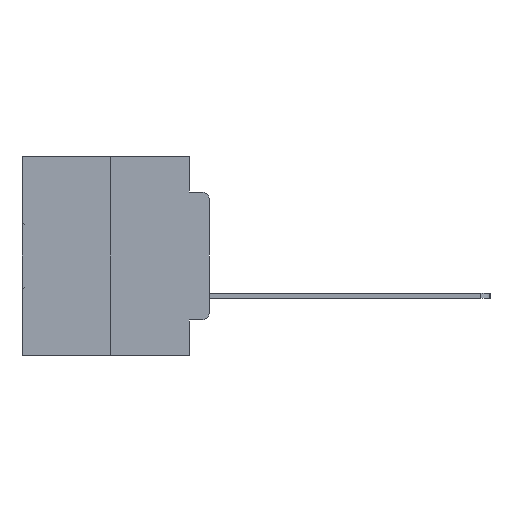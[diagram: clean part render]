
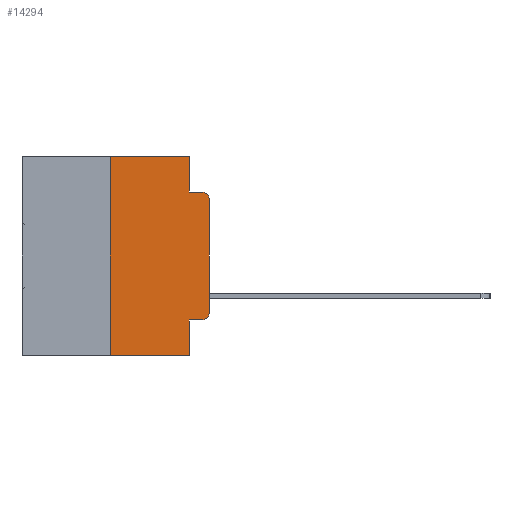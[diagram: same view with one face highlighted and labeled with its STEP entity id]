
A CAD part, left-side view. The second image highlights one B-rep face of the part: STEP entity #14294.
In plain terms, the highlighted planar face has unit normal (-1, 0, 0).
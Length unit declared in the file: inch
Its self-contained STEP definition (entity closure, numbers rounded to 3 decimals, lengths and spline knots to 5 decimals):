
#706 = ORIENTED_EDGE ( 'NONE', *, *, #26774, .F. ) ;
#952 = DIRECTION ( 'NONE',  ( 1., 0., 0. ) ) ;
#971 = LINE ( 'NONE', #20506, #6593 ) ;
#1657 = CARTESIAN_POINT ( 'NONE',  ( 0., 0.25, -0.5 ) ) ;
#2181 = ORIENTED_EDGE ( 'NONE', *, *, #8467, .T. ) ;
#2352 = LINE ( 'NONE', #14920, #7245 ) ;
#2568 = CARTESIAN_POINT ( 'NONE',  ( 0., 0.051, -0.0885 ) ) ;
#2713 = DIRECTION ( 'NONE',  ( -1., 0., 0. ) ) ;
#2879 = CARTESIAN_POINT ( 'NONE',  ( 0., 0., -0.3915 ) ) ;
#4045 = ORIENTED_EDGE ( 'NONE', *, *, #10219, .F. ) ;
#5011 = LINE ( 'NONE', #5101, #28665 ) ;
#5101 = CARTESIAN_POINT ( 'NONE',  ( 0., 0.051, 0. ) ) ;
#5233 = CARTESIAN_POINT ( 'NONE',  ( 0., 0.051, -0.4115 ) ) ;
#5458 = CARTESIAN_POINT ( 'NONE',  ( 0., 0.25, 0. ) ) ;
#6114 = VECTOR ( 'NONE', #24786, 39.37008 ) ;
#6127 = CARTESIAN_POINT ( 'NONE',  ( 0., 0.051, -0.5 ) ) ;
#6136 = CARTESIAN_POINT ( 'NONE',  ( 0., 0., -0.1085 ) ) ;
#6593 = VECTOR ( 'NONE', #22897, 39.37008 ) ;
#7245 = VECTOR ( 'NONE', #17186, 39.37008 ) ;
#7883 = DIRECTION ( 'NONE',  ( 0., 0., 1. ) ) ;
#8215 = VERTEX_POINT ( 'NONE', #1657 ) ;
#8255 = VERTEX_POINT ( 'NONE', #9101 ) ;
#8276 = VERTEX_POINT ( 'NONE', #27923 ) ;
#8467 = EDGE_CURVE ( 'NONE', #8215, #18024, #19952, .T. ) ;
#8807 = CIRCLE ( 'NONE', #24011, 0.02 ) ;
#8814 = CARTESIAN_POINT ( 'NONE',  ( 0., 0.473, 0. ) ) ;
#9101 = CARTESIAN_POINT ( 'NONE',  ( 0., 0.02, -0.0885 ) ) ;
#9537 = VECTOR ( 'NONE', #25926, 39.37008 ) ;
#10219 = EDGE_CURVE ( 'NONE', #8276, #28659, #19099, .T. ) ;
#11506 = DIRECTION ( 'NONE',  ( 0., -1., 0. ) ) ;
#12866 = CARTESIAN_POINT ( 'NONE',  ( 0., 0.473, 0. ) ) ;
#13652 = CARTESIAN_POINT ( 'NONE',  ( 0., 0.02, -0.1085 ) ) ;
#13888 = VERTEX_POINT ( 'NONE', #6136 ) ;
#13963 = LINE ( 'NONE', #17682, #6114 ) ;
#14103 = CARTESIAN_POINT ( 'NONE',  ( 0., 0.051, 0. ) ) ;
#14232 = VERTEX_POINT ( 'NONE', #26643 ) ;
#14294 = ADVANCED_FACE ( 'NONE', ( #25542 ), #22254, .F. ) ;
#14920 = CARTESIAN_POINT ( 'NONE',  ( 0., 0.051, -0.0885 ) ) ;
#15643 = EDGE_CURVE ( 'NONE', #21927, #14232, #971, .T. ) ;
#15954 = AXIS2_PLACEMENT_3D ( 'NONE', #12866, #952, #17613 ) ;
#15991 = ORIENTED_EDGE ( 'NONE', *, *, #20480, .F. ) ;
#16011 = DIRECTION ( 'NONE',  ( 0., 0., -1. ) ) ;
#16371 = ORIENTED_EDGE ( 'NONE', *, *, #16571, .F. ) ;
#16571 = EDGE_CURVE ( 'NONE', #21927, #18024, #5011, .T. ) ;
#16829 = CARTESIAN_POINT ( 'NONE',  ( 0., 0.051, 0. ) ) ;
#16968 = DIRECTION ( 'NONE',  ( 0., 0., -1. ) ) ;
#16992 = CARTESIAN_POINT ( 'NONE',  ( 0., 0.02, -0.3915 ) ) ;
#17083 = ORIENTED_EDGE ( 'NONE', *, *, #20782, .T. ) ;
#17186 = DIRECTION ( 'NONE',  ( 0., -1., 0. ) ) ;
#17613 = DIRECTION ( 'NONE',  ( 0., 0., -1. ) ) ;
#17682 = CARTESIAN_POINT ( 'NONE',  ( 0., 0., 0. ) ) ;
#17763 = VERTEX_POINT ( 'NONE', #2568 ) ;
#18024 = VERTEX_POINT ( 'NONE', #6127 ) ;
#18377 = VECTOR ( 'NONE', #23060, 39.37008 ) ;
#19099 = LINE ( 'NONE', #8814, #18377 ) ;
#19323 = DIRECTION ( 'NONE',  ( 0., 0., -1. ) ) ;
#19952 = LINE ( 'NONE', #27935, #25493 ) ;
#20086 = EDGE_CURVE ( 'NONE', #14232, #26075, #8807, .T. ) ;
#20480 = EDGE_CURVE ( 'NONE', #28659, #17763, #22828, .T. ) ;
#20506 = CARTESIAN_POINT ( 'NONE',  ( 0., 0.051, -0.4115 ) ) ;
#20751 = ORIENTED_EDGE ( 'NONE', *, *, #27347, .F. ) ;
#20782 = EDGE_CURVE ( 'NONE', #26075, #13888, #13963, .T. ) ;
#21257 = AXIS2_PLACEMENT_3D ( 'NONE', #13652, #30038, #16011 ) ;
#21927 = VERTEX_POINT ( 'NONE', #5233 ) ;
#22254 = PLANE ( 'NONE',  #15954 ) ;
#22274 = EDGE_LOOP ( 'NONE', ( #17083, #25544, #20751, #15991, #4045, #706, #2181, #16371, #28838, #25575 ) ) ;
#22631 = CIRCLE ( 'NONE', #21257, 0.02 ) ;
#22828 = LINE ( 'NONE', #14103, #9537 ) ;
#22897 = DIRECTION ( 'NONE',  ( 0., -1., 0. ) ) ;
#23060 = DIRECTION ( 'NONE',  ( 0., -1., 0. ) ) ;
#24011 = AXIS2_PLACEMENT_3D ( 'NONE', #16992, #2713, #19323 ) ;
#24313 = VECTOR ( 'NONE', #7883, 39.37008 ) ;
#24786 = DIRECTION ( 'NONE',  ( 0., 0., 1. ) ) ;
#25044 = LINE ( 'NONE', #5458, #24313 ) ;
#25493 = VECTOR ( 'NONE', #11506, 39.37008 ) ;
#25542 = FACE_OUTER_BOUND ( 'NONE', #22274, .T. ) ;
#25544 = ORIENTED_EDGE ( 'NONE', *, *, #30339, .T. ) ;
#25575 = ORIENTED_EDGE ( 'NONE', *, *, #20086, .T. ) ;
#25926 = DIRECTION ( 'NONE',  ( 0., 0., -1. ) ) ;
#26075 = VERTEX_POINT ( 'NONE', #2879 ) ;
#26643 = CARTESIAN_POINT ( 'NONE',  ( 0., 0.02, -0.4115 ) ) ;
#26774 = EDGE_CURVE ( 'NONE', #8215, #8276, #25044, .T. ) ;
#27347 = EDGE_CURVE ( 'NONE', #17763, #8255, #2352, .T. ) ;
#27923 = CARTESIAN_POINT ( 'NONE',  ( 0., 0.25, 0. ) ) ;
#27935 = CARTESIAN_POINT ( 'NONE',  ( 0., 0.473, -0.5 ) ) ;
#28659 = VERTEX_POINT ( 'NONE', #16829 ) ;
#28665 = VECTOR ( 'NONE', #16968, 39.37008 ) ;
#28838 = ORIENTED_EDGE ( 'NONE', *, *, #15643, .T. ) ;
#30038 = DIRECTION ( 'NONE',  ( -1., 0., 0. ) ) ;
#30339 = EDGE_CURVE ( 'NONE', #13888, #8255, #22631, .T. ) ;
